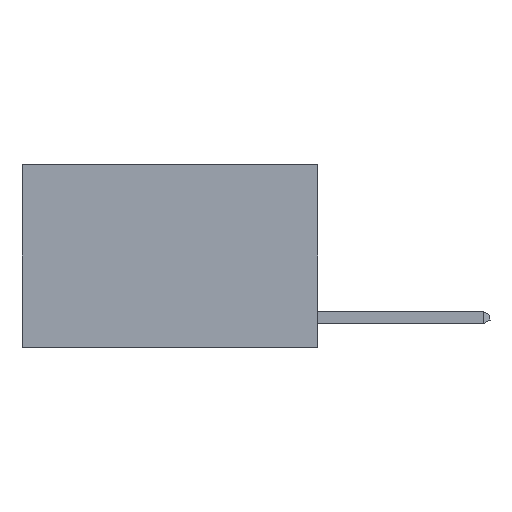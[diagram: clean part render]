
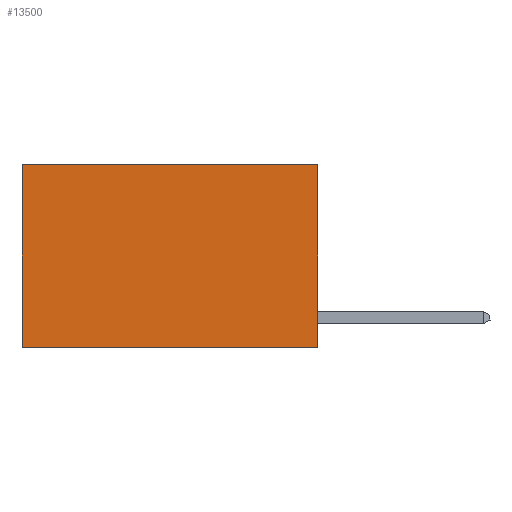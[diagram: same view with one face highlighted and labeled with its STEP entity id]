
A CAD part, left-side view. The second image highlights one B-rep face of the part: STEP entity #13500.
In plain terms, the highlighted planar face has unit normal (-1, 0, 0).
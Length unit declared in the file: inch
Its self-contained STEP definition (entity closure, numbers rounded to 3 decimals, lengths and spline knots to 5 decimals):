
#13 = DIRECTION ( 'NONE',  ( 1., 0., 0. ) ) ;
#39 = VECTOR ( 'NONE', #10499, 39.37008 ) ;
#524 = CARTESIAN_POINT ( 'NONE',  ( 0.2625, 0.6, -0.37 ) ) ;
#836 = CARTESIAN_POINT ( 'NONE',  ( 0.2625, 0., 0. ) ) ;
#1526 = LINE ( 'NONE', #19461, #14200 ) ;
#3836 = VECTOR ( 'NONE', #19621, 39.37008 ) ;
#4905 = PLANE ( 'NONE',  #10818 ) ;
#5202 = LINE ( 'NONE', #6175, #16855 ) ;
#6175 = CARTESIAN_POINT ( 'NONE',  ( 0.2625, 0., -0.37 ) ) ;
#7701 = LINE ( 'NONE', #836, #39 ) ;
#7776 = DIRECTION ( 'NONE',  ( 0., 1., 0. ) ) ;
#9727 = CARTESIAN_POINT ( 'NONE',  ( 0.2625, 0., 0. ) ) ;
#9848 = ORIENTED_EDGE ( 'NONE', *, *, #12184, .F. ) ;
#10233 = DIRECTION ( 'NONE',  ( 0., 0., -1. ) ) ;
#10499 = DIRECTION ( 'NONE',  ( 0., 0., -1. ) ) ;
#10818 = AXIS2_PLACEMENT_3D ( 'NONE', #9727, #13, #11278 ) ;
#10910 = CARTESIAN_POINT ( 'NONE',  ( 0.2625, 0.6, 0. ) ) ;
#11221 = VERTEX_POINT ( 'NONE', #524 ) ;
#11278 = DIRECTION ( 'NONE',  ( 0., 0., -1. ) ) ;
#11721 = VERTEX_POINT ( 'NONE', #14373 ) ;
#12184 = EDGE_CURVE ( 'NONE', #11721, #11221, #5202, .T. ) ;
#12515 = EDGE_CURVE ( 'NONE', #19476, #11221, #1526, .T. ) ;
#13500 = ADVANCED_FACE ( 'NONE', ( #14859 ), #4905, .F. ) ;
#13695 = ORIENTED_EDGE ( 'NONE', *, *, #19273, .T. ) ;
#14081 = LINE ( 'NONE', #19686, #3836 ) ;
#14200 = VECTOR ( 'NONE', #10233, 39.37008 ) ;
#14373 = CARTESIAN_POINT ( 'NONE',  ( 0.2625, 0., -0.37 ) ) ;
#14859 = FACE_OUTER_BOUND ( 'NONE', #14991, .T. ) ;
#14991 = EDGE_LOOP ( 'NONE', ( #19151, #9848, #18868, #13695 ) ) ;
#16855 = VECTOR ( 'NONE', #7776, 39.37008 ) ;
#17185 = CARTESIAN_POINT ( 'NONE',  ( 0.2625, 0., 0. ) ) ;
#17996 = EDGE_CURVE ( 'NONE', #18887, #11721, #7701, .T. ) ;
#18868 = ORIENTED_EDGE ( 'NONE', *, *, #17996, .F. ) ;
#18887 = VERTEX_POINT ( 'NONE', #17185 ) ;
#19151 = ORIENTED_EDGE ( 'NONE', *, *, #12515, .T. ) ;
#19273 = EDGE_CURVE ( 'NONE', #18887, #19476, #14081, .T. ) ;
#19461 = CARTESIAN_POINT ( 'NONE',  ( 0.2625, 0.6, 0. ) ) ;
#19476 = VERTEX_POINT ( 'NONE', #10910 ) ;
#19621 = DIRECTION ( 'NONE',  ( 0., 1., 0. ) ) ;
#19686 = CARTESIAN_POINT ( 'NONE',  ( 0.2625, 0., 0. ) ) ;
